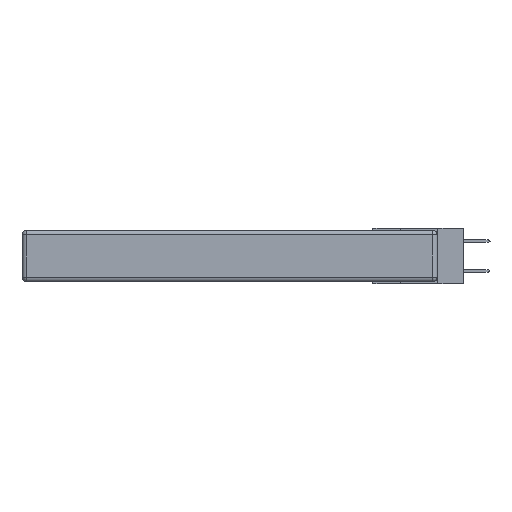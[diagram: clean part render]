
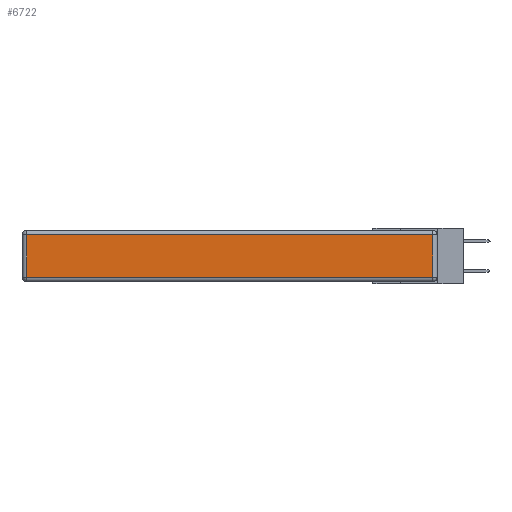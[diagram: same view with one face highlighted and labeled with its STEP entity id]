
A CAD part, left-side view. The second image highlights one B-rep face of the part: STEP entity #6722.
In plain terms, the highlighted planar face has unit normal (-1, 0, 0).
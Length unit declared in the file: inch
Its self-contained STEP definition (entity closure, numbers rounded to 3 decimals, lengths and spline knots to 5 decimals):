
#822 = EDGE_CURVE ( 'NONE', #10329, #3075, #3239, .T. ) ;
#1022 = LINE ( 'NONE', #11915, #13232 ) ;
#1111 = CARTESIAN_POINT ( 'NONE',  ( 0., 0.03, -0.03 ) ) ;
#1636 = ORIENTED_EDGE ( 'NONE', *, *, #822, .T. ) ;
#1652 = AXIS2_PLACEMENT_3D ( 'NONE', #16881, #8795, #18454 ) ;
#1757 = VECTOR ( 'NONE', #6730, 39.37008 ) ;
#2566 = ORIENTED_EDGE ( 'NONE', *, *, #6780, .T. ) ;
#2881 = LINE ( 'NONE', #6372, #6832 ) ;
#3075 = VERTEX_POINT ( 'NONE', #17988 ) ;
#3239 = LINE ( 'NONE', #13129, #1757 ) ;
#4270 = PLANE ( 'NONE',  #1652 ) ;
#4776 = DIRECTION ( 'NONE',  ( 0., 0., -1. ) ) ;
#5533 = DIRECTION ( 'NONE',  ( 0., 0., 1. ) ) ;
#6372 = CARTESIAN_POINT ( 'NONE',  ( 0., 2.72, -0.343 ) ) ;
#6722 = ADVANCED_FACE ( 'NONE', ( #18397 ), #4270, .T. ) ;
#6730 = DIRECTION ( 'NONE',  ( 0., 1., 0. ) ) ;
#6773 = ORIENTED_EDGE ( 'NONE', *, *, #11078, .T. ) ;
#6780 = EDGE_CURVE ( 'NONE', #20169, #12794, #14943, .T. ) ;
#6832 = VECTOR ( 'NONE', #4776, 39.37008 ) ;
#8795 = DIRECTION ( 'NONE',  ( -1., 0., 0. ) ) ;
#9119 = EDGE_LOOP ( 'NONE', ( #2566, #16157, #1636, #6773 ) ) ;
#10063 = CARTESIAN_POINT ( 'NONE',  ( 0., 2.72, -0.313 ) ) ;
#10329 = VERTEX_POINT ( 'NONE', #1111 ) ;
#10971 = DIRECTION ( 'NONE',  ( 0., -1., 0. ) ) ;
#11078 = EDGE_CURVE ( 'NONE', #3075, #20169, #2881, .T. ) ;
#11915 = CARTESIAN_POINT ( 'NONE',  ( 0., 0.03, -0.343 ) ) ;
#12794 = VERTEX_POINT ( 'NONE', #13400 ) ;
#13129 = CARTESIAN_POINT ( 'NONE',  ( 0., 2.75, -0.03 ) ) ;
#13232 = VECTOR ( 'NONE', #5533, 39.37008 ) ;
#13400 = CARTESIAN_POINT ( 'NONE',  ( 0., 0.03, -0.313 ) ) ;
#14068 = EDGE_CURVE ( 'NONE', #12794, #10329, #1022, .T. ) ;
#14943 = LINE ( 'NONE', #17288, #19740 ) ;
#16157 = ORIENTED_EDGE ( 'NONE', *, *, #14068, .T. ) ;
#16881 = CARTESIAN_POINT ( 'NONE',  ( 0., 0., -0.343 ) ) ;
#17288 = CARTESIAN_POINT ( 'NONE',  ( 0., 0., -0.313 ) ) ;
#17988 = CARTESIAN_POINT ( 'NONE',  ( 0., 2.72, -0.03 ) ) ;
#18397 = FACE_OUTER_BOUND ( 'NONE', #9119, .T. ) ;
#18454 = DIRECTION ( 'NONE',  ( 0., 0., 1. ) ) ;
#19740 = VECTOR ( 'NONE', #10971, 39.37008 ) ;
#20169 = VERTEX_POINT ( 'NONE', #10063 ) ;
